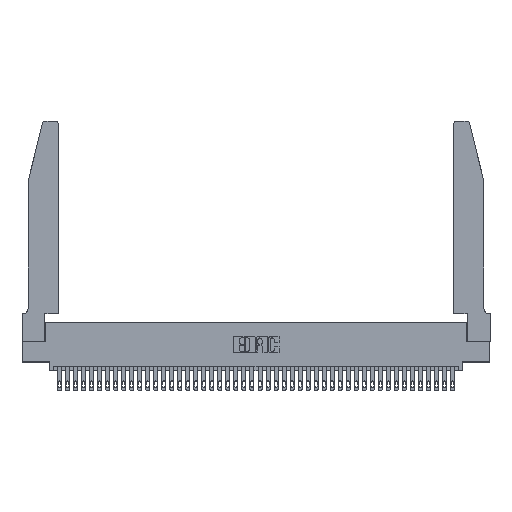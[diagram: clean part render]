
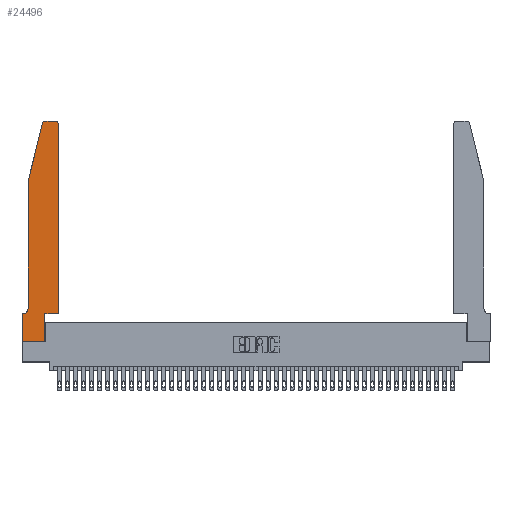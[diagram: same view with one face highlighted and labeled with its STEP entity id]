
A CAD part, top view. The second image highlights one B-rep face of the part: STEP entity #24496.
In plain terms, the highlighted planar face has unit normal (0, 0, 1).
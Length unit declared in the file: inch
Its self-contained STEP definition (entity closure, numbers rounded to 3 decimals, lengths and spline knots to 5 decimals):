
#9 = CARTESIAN_POINT ( 'NONE',  ( 0., 0., 0.37 ) ) ;
#934 = EDGE_CURVE ( 'NONE', #40589, #34033, #23681, .T. ) ;
#1082 = CARTESIAN_POINT ( 'NONE',  ( 0.4505, 0.35, 0.37 ) ) ;
#1384 = CARTESIAN_POINT ( 'NONE',  ( 0.0755, 2., 0.37 ) ) ;
#1789 = DIRECTION ( 'NONE',  ( 0., 0., 1. ) ) ;
#2014 = EDGE_CURVE ( 'NONE', #42400, #34261, #20646, .T. ) ;
#2781 = ORIENTED_EDGE ( 'NONE', *, *, #39813, .T. ) ;
#3023 = CARTESIAN_POINT ( 'NONE',  ( 0.0055, 0.35, 0.37 ) ) ;
#3132 = CIRCLE ( 'NONE', #8658, 0.03 ) ;
#3661 = ORIENTED_EDGE ( 'NONE', *, *, #20782, .T. ) ;
#3959 = EDGE_CURVE ( 'NONE', #40565, #40589, #37557, .T. ) ;
#4606 = LINE ( 'NONE', #4673, #27509 ) ;
#4673 = CARTESIAN_POINT ( 'NONE',  ( 0.2605, 2.75, 0.37 ) ) ;
#5423 = DIRECTION ( 'NONE',  ( 1., 0., 0. ) ) ;
#8391 = CARTESIAN_POINT ( 'NONE',  ( 0.4505, 0.35, 0.37 ) ) ;
#8501 = DIRECTION ( 'NONE',  ( 0., 0., 1. ) ) ;
#8658 = AXIS2_PLACEMENT_3D ( 'NONE', #32905, #39175, #23087 ) ;
#8943 = LINE ( 'NONE', #9, #41655 ) ;
#9229 = VERTEX_POINT ( 'NONE', #3023 ) ;
#10510 = VECTOR ( 'NONE', #40708, 39.37008 ) ;
#10680 = CARTESIAN_POINT ( 'NONE',  ( 0.0755, 2., 0.37 ) ) ;
#11125 = EDGE_CURVE ( 'NONE', #11225, #9229, #30137, .T. ) ;
#11225 = VERTEX_POINT ( 'NONE', #41580 ) ;
#11339 = LINE ( 'NONE', #34795, #14966 ) ;
#11499 = ORIENTED_EDGE ( 'NONE', *, *, #25022, .T. ) ;
#11595 = ORIENTED_EDGE ( 'NONE', *, *, #26985, .T. ) ;
#11699 = DIRECTION ( 'NONE',  ( 0., 1., 0. ) ) ;
#11708 = CARTESIAN_POINT ( 'NONE',  ( 0.4505, 2.72, 0.37 ) ) ;
#12186 = ORIENTED_EDGE ( 'NONE', *, *, #934, .T. ) ;
#12383 = DIRECTION ( 'NONE',  ( 0., 1., 0. ) ) ;
#12598 = CIRCLE ( 'NONE', #21624, 0.03 ) ;
#14389 = DIRECTION ( 'NONE',  ( -1., 0., 0. ) ) ;
#14966 = VECTOR ( 'NONE', #31497, 39.37008 ) ;
#15819 = DIRECTION ( 'NONE',  ( -1., 0., 0. ) ) ;
#16391 = DIRECTION ( 'NONE',  ( 1., 0., 0. ) ) ;
#16618 = DIRECTION ( 'NONE',  ( -0.239, -0.971, 0. ) ) ;
#17081 = VECTOR ( 'NONE', #14389, 39.37008 ) ;
#17348 = CARTESIAN_POINT ( 'NONE',  ( 0., 0.35, 0.37 ) ) ;
#17779 = EDGE_CURVE ( 'NONE', #42033, #42400, #12598, .T. ) ;
#18449 = DIRECTION ( 'NONE',  ( 1., 0., 0. ) ) ;
#18629 = LINE ( 'NONE', #34839, #17081 ) ;
#18808 = ORIENTED_EDGE ( 'NONE', *, *, #11125, .T. ) ;
#19085 = DIRECTION ( 'NONE',  ( 1., 0., 0. ) ) ;
#19231 = AXIS2_PLACEMENT_3D ( 'NONE', #31985, #8501, #5423 ) ;
#19439 = VERTEX_POINT ( 'NONE', #17348 ) ;
#20646 = LINE ( 'NONE', #10680, #39349 ) ;
#20782 = EDGE_CURVE ( 'NONE', #19439, #26489, #11339, .T. ) ;
#20852 = EDGE_CURVE ( 'NONE', #33736, #40565, #31604, .T. ) ;
#20984 = CARTESIAN_POINT ( 'NONE',  ( 0.2865, 0.35, 0.37 ) ) ;
#21624 = AXIS2_PLACEMENT_3D ( 'NONE', #21670, #1789, #18449 ) ;
#21670 = CARTESIAN_POINT ( 'NONE',  ( 0.284, 2.72, 0.37 ) ) ;
#23087 = DIRECTION ( 'NONE',  ( 1., 0., 0. ) ) ;
#23663 = ORIENTED_EDGE ( 'NONE', *, *, #2014, .T. ) ;
#23681 = LINE ( 'NONE', #8391, #35105 ) ;
#23779 = CARTESIAN_POINT ( 'NONE',  ( 0.25487, 2.72718, 0.37 ) ) ;
#24327 = CARTESIAN_POINT ( 'NONE',  ( 0.2865, 0.35, 0.37 ) ) ;
#24496 = ADVANCED_FACE ( 'NONE', ( #28769 ), #28950, .T. ) ;
#24584 = DIRECTION ( 'NONE',  ( -1., 0., 0. ) ) ;
#25022 = EDGE_CURVE ( 'NONE', #34261, #11225, #28239, .T. ) ;
#25370 = AXIS2_PLACEMENT_3D ( 'NONE', #35709, #29371, #15819 ) ;
#26489 = VERTEX_POINT ( 'NONE', #27361 ) ;
#26985 = EDGE_CURVE ( 'NONE', #9229, #19439, #18629, .T. ) ;
#26999 = EDGE_CURVE ( 'NONE', #36143, #42033, #4606, .T. ) ;
#27361 = CARTESIAN_POINT ( 'NONE',  ( 0., 0., 0.37 ) ) ;
#27405 = CARTESIAN_POINT ( 'NONE',  ( 0.4205, 2.75, 0.37 ) ) ;
#27469 = CARTESIAN_POINT ( 'NONE',  ( 0.4505, 0.35, 0.37 ) ) ;
#27509 = VECTOR ( 'NONE', #24584, 39.37008 ) ;
#27973 = ORIENTED_EDGE ( 'NONE', *, *, #20852, .T. ) ;
#28239 = LINE ( 'NONE', #1384, #10510 ) ;
#28769 = FACE_OUTER_BOUND ( 'NONE', #35987, .T. ) ;
#28950 = PLANE ( 'NONE',  #19231 ) ;
#29348 = ORIENTED_EDGE ( 'NONE', *, *, #26999, .T. ) ;
#29371 = DIRECTION ( 'NONE',  ( 0., 0., -1. ) ) ;
#30137 = CIRCLE ( 'NONE', #25370, 0.07 ) ;
#31497 = DIRECTION ( 'NONE',  ( 0., -1., 0. ) ) ;
#31604 = LINE ( 'NONE', #24327, #39376 ) ;
#31985 = CARTESIAN_POINT ( 'NONE',  ( 0., 0.35, 0.37 ) ) ;
#32905 = CARTESIAN_POINT ( 'NONE',  ( 0.4205, 2.72, 0.37 ) ) ;
#32917 = ORIENTED_EDGE ( 'NONE', *, *, #3959, .T. ) ;
#32992 = CARTESIAN_POINT ( 'NONE',  ( 0.0755, 2., 0.37 ) ) ;
#33278 = ORIENTED_EDGE ( 'NONE', *, *, #17779, .T. ) ;
#33736 = VERTEX_POINT ( 'NONE', #33749 ) ;
#33749 = CARTESIAN_POINT ( 'NONE',  ( 0.2865, 0., 0.37 ) ) ;
#34033 = VERTEX_POINT ( 'NONE', #11708 ) ;
#34261 = VERTEX_POINT ( 'NONE', #32992 ) ;
#34795 = CARTESIAN_POINT ( 'NONE',  ( 0., 0., 0.37 ) ) ;
#34839 = CARTESIAN_POINT ( 'NONE',  ( 0.0755, 0.35, 0.37 ) ) ;
#35105 = VECTOR ( 'NONE', #11699, 39.37008 ) ;
#35340 = EDGE_CURVE ( 'NONE', #34033, #36143, #3132, .T. ) ;
#35709 = CARTESIAN_POINT ( 'NONE',  ( 0.0055, 0.42, 0.37 ) ) ;
#35931 = ORIENTED_EDGE ( 'NONE', *, *, #35340, .T. ) ;
#35987 = EDGE_LOOP ( 'NONE', ( #29348, #33278, #23663, #11499, #18808, #11595, #3661, #2781, #27973, #32917, #12186, #35931 ) ) ;
#36143 = VERTEX_POINT ( 'NONE', #27405 ) ;
#37557 = LINE ( 'NONE', #27469, #38638 ) ;
#38638 = VECTOR ( 'NONE', #19085, 39.37008 ) ;
#39175 = DIRECTION ( 'NONE',  ( 0., 0., 1. ) ) ;
#39349 = VECTOR ( 'NONE', #16618, 39.37008 ) ;
#39376 = VECTOR ( 'NONE', #12383, 39.37008 ) ;
#39813 = EDGE_CURVE ( 'NONE', #26489, #33736, #8943, .T. ) ;
#40565 = VERTEX_POINT ( 'NONE', #20984 ) ;
#40589 = VERTEX_POINT ( 'NONE', #1082 ) ;
#40708 = DIRECTION ( 'NONE',  ( 0., -1., 0. ) ) ;
#41580 = CARTESIAN_POINT ( 'NONE',  ( 0.0755, 0.42, 0.37 ) ) ;
#41655 = VECTOR ( 'NONE', #16391, 39.37008 ) ;
#42033 = VERTEX_POINT ( 'NONE', #42094 ) ;
#42094 = CARTESIAN_POINT ( 'NONE',  ( 0.284, 2.75, 0.37 ) ) ;
#42400 = VERTEX_POINT ( 'NONE', #23779 ) ;
